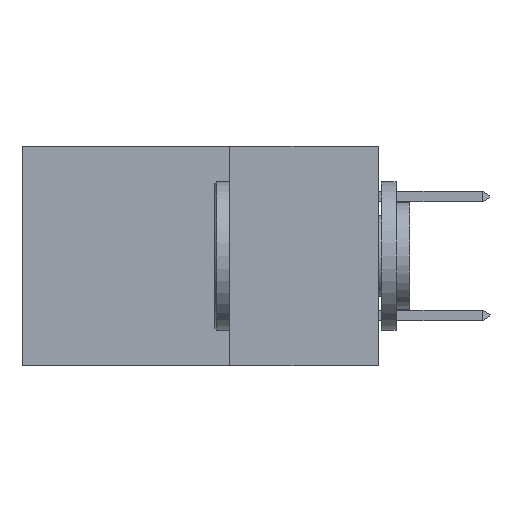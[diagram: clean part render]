
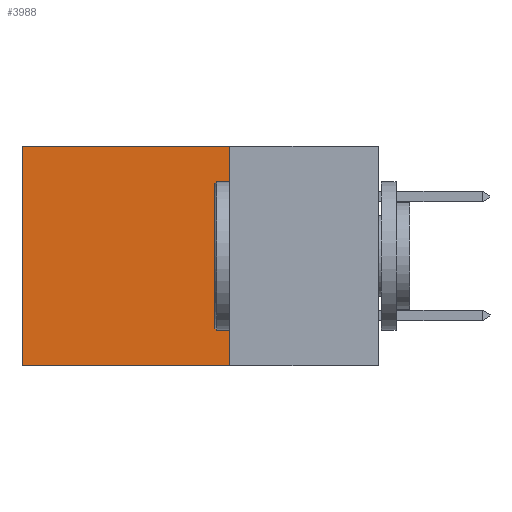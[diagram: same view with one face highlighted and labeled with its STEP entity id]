
A CAD part, left-side view. The second image highlights one B-rep face of the part: STEP entity #3988.
In plain terms, the highlighted planar face has unit normal (-1, 0, 0).
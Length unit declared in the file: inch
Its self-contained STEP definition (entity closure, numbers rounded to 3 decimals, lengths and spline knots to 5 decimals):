
#382 = EDGE_LOOP ( 'NONE', ( #981, #12451, #8321, #11401 ) ) ;
#616 = VERTEX_POINT ( 'NONE', #10600 ) ;
#967 = DIRECTION ( 'NONE',  ( 1., 0., 0. ) ) ;
#981 = ORIENTED_EDGE ( 'NONE', *, *, #3425, .T. ) ;
#1110 = EDGE_CURVE ( 'NONE', #11547, #1546, #7639, .T. ) ;
#1281 = DIRECTION ( 'NONE',  ( 0., 1., 0. ) ) ;
#1546 = VERTEX_POINT ( 'NONE', #4053 ) ;
#1820 = DIRECTION ( 'NONE',  ( 0., 0., -1. ) ) ;
#1839 = LINE ( 'NONE', #5445, #12487 ) ;
#3138 = FACE_OUTER_BOUND ( 'NONE', #382, .T. ) ;
#3405 = DIRECTION ( 'NONE',  ( 0., 0., -1. ) ) ;
#3425 = EDGE_CURVE ( 'NONE', #4407, #616, #11833, .T. ) ;
#3537 = CARTESIAN_POINT ( 'NONE',  ( 0.298, 0.6, 0. ) ) ;
#3630 = EDGE_CURVE ( 'NONE', #11547, #4407, #7955, .T. ) ;
#3777 = VECTOR ( 'NONE', #4456, 39.37008 ) ;
#3988 = ADVANCED_FACE ( 'NONE', ( #3138 ), #10241, .F. ) ;
#4053 = CARTESIAN_POINT ( 'NONE',  ( 0.298, 0.25, -0.37 ) ) ;
#4407 = VERTEX_POINT ( 'NONE', #8114 ) ;
#4456 = DIRECTION ( 'NONE',  ( 0., 0., -1. ) ) ;
#5182 = AXIS2_PLACEMENT_3D ( 'NONE', #13243, #967, #1820 ) ;
#5445 = CARTESIAN_POINT ( 'NONE',  ( 0.298, 0.25, -0.37 ) ) ;
#7326 = VECTOR ( 'NONE', #11271, 39.37008 ) ;
#7590 = CARTESIAN_POINT ( 'NONE',  ( 0.298, 0.25, 0. ) ) ;
#7639 = LINE ( 'NONE', #7590, #3777 ) ;
#7955 = LINE ( 'NONE', #10358, #7326 ) ;
#8114 = CARTESIAN_POINT ( 'NONE',  ( 0.298, 0.6, 0. ) ) ;
#8321 = ORIENTED_EDGE ( 'NONE', *, *, #1110, .F. ) ;
#10241 = PLANE ( 'NONE',  #5182 ) ;
#10358 = CARTESIAN_POINT ( 'NONE',  ( 0.298, 0.25, 0. ) ) ;
#10600 = CARTESIAN_POINT ( 'NONE',  ( 0.298, 0.6, -0.37 ) ) ;
#11025 = VECTOR ( 'NONE', #3405, 39.37008 ) ;
#11271 = DIRECTION ( 'NONE',  ( 0., 1., 0. ) ) ;
#11401 = ORIENTED_EDGE ( 'NONE', *, *, #3630, .T. ) ;
#11482 = EDGE_CURVE ( 'NONE', #1546, #616, #1839, .T. ) ;
#11547 = VERTEX_POINT ( 'NONE', #12790 ) ;
#11833 = LINE ( 'NONE', #3537, #11025 ) ;
#12451 = ORIENTED_EDGE ( 'NONE', *, *, #11482, .F. ) ;
#12487 = VECTOR ( 'NONE', #1281, 39.37008 ) ;
#12790 = CARTESIAN_POINT ( 'NONE',  ( 0.298, 0.25, 0. ) ) ;
#13243 = CARTESIAN_POINT ( 'NONE',  ( 0.298, 0.25, 0. ) ) ;
